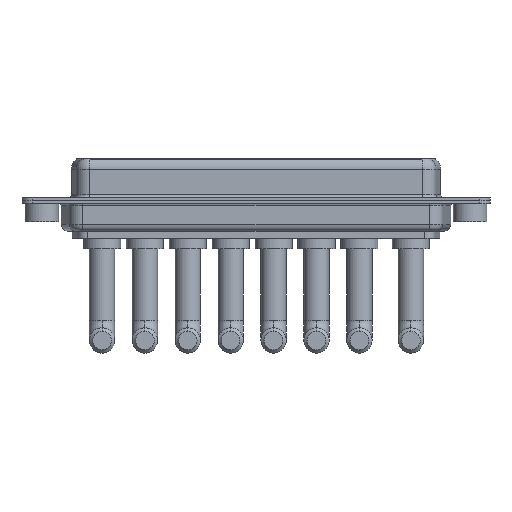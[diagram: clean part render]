
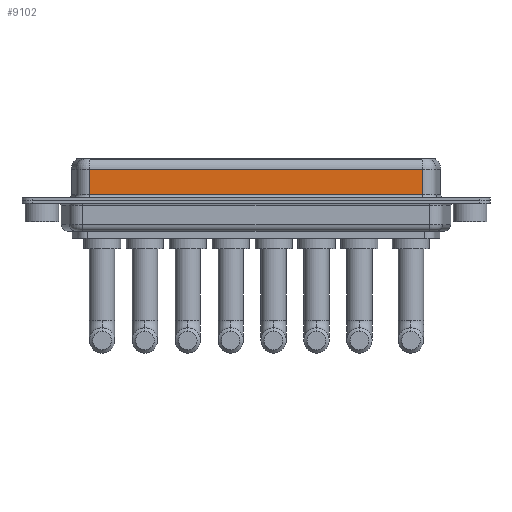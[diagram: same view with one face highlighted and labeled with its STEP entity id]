
A CAD part, front view. The second image highlights one B-rep face of the part: STEP entity #9102.
In plain terms, the highlighted planar face has unit normal (0, -1, 0).
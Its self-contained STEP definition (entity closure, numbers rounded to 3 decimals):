
#228 = ORIENTED_EDGE ( 'NONE', *, *, #5265, .T. ) ;
#449 = DIRECTION ( 'NONE',  ( 0., 0., 1. ) ) ;
#937 = CARTESIAN_POINT ( 'NONE',  ( 56.462, -3.95, 4.65 ) ) ;
#2151 = ORIENTED_EDGE ( 'NONE', *, *, #2552, .T. ) ;
#2213 = VECTOR ( 'NONE', #11408, 1000. ) ;
#2552 = EDGE_CURVE ( 'NONE', #7472, #10362, #9598, .T. ) ;
#3455 = VECTOR ( 'NONE', #10033, 1000. ) ;
#4029 = CARTESIAN_POINT ( 'NONE',  ( 56.462, -3.95, 0.9 ) ) ;
#4274 = AXIS2_PLACEMENT_3D ( 'NONE', #7142, #11243, #449 ) ;
#4376 = FACE_OUTER_BOUND ( 'NONE', #8715, .T. ) ;
#4445 = EDGE_CURVE ( 'NONE', #10744, #6502, #7120, .T. ) ;
#5265 = EDGE_CURVE ( 'NONE', #10744, #7472, #12204, .T. ) ;
#5550 = CARTESIAN_POINT ( 'NONE',  ( 7.038, -3.95, 6.4 ) ) ;
#5896 = CARTESIAN_POINT ( 'NONE',  ( 56.462, -3.95, 6.4 ) ) ;
#6502 = VERTEX_POINT ( 'NONE', #12021 ) ;
#7120 = LINE ( 'NONE', #5896, #9153 ) ;
#7142 = CARTESIAN_POINT ( 'NONE',  ( 56.462, -3.95, 6.4 ) ) ;
#7472 = VERTEX_POINT ( 'NONE', #8830 ) ;
#7844 = CARTESIAN_POINT ( 'NONE',  ( 7.038, -3.95, 0.9 ) ) ;
#7954 = LINE ( 'NONE', #4029, #3455 ) ;
#8715 = EDGE_LOOP ( 'NONE', ( #11271, #228, #2151, #10174 ) ) ;
#8830 = CARTESIAN_POINT ( 'NONE',  ( 7.038, -3.95, 4.65 ) ) ;
#9102 = ADVANCED_FACE ( 'NONE', ( #4376 ), #12581, .F. ) ;
#9153 = VECTOR ( 'NONE', #13029, 1000. ) ;
#9241 = CARTESIAN_POINT ( 'NONE',  ( 56.462, -3.95, 4.65 ) ) ;
#9598 = LINE ( 'NONE', #5550, #2213 ) ;
#10033 = DIRECTION ( 'NONE',  ( 1., 0., 0. ) ) ;
#10174 = ORIENTED_EDGE ( 'NONE', *, *, #11759, .T. ) ;
#10362 = VERTEX_POINT ( 'NONE', #7844 ) ;
#10744 = VERTEX_POINT ( 'NONE', #937 ) ;
#11061 = DIRECTION ( 'NONE',  ( -1., 0., 0. ) ) ;
#11243 = DIRECTION ( 'NONE',  ( 0., 1., 0. ) ) ;
#11271 = ORIENTED_EDGE ( 'NONE', *, *, #4445, .F. ) ;
#11408 = DIRECTION ( 'NONE',  ( 0., 0., -1. ) ) ;
#11759 = EDGE_CURVE ( 'NONE', #10362, #6502, #7954, .T. ) ;
#11955 = VECTOR ( 'NONE', #11061, 1000. ) ;
#12021 = CARTESIAN_POINT ( 'NONE',  ( 56.462, -3.95, 0.9 ) ) ;
#12204 = LINE ( 'NONE', #9241, #11955 ) ;
#12581 = PLANE ( 'NONE',  #4274 ) ;
#13029 = DIRECTION ( 'NONE',  ( 0., 0., -1. ) ) ;
